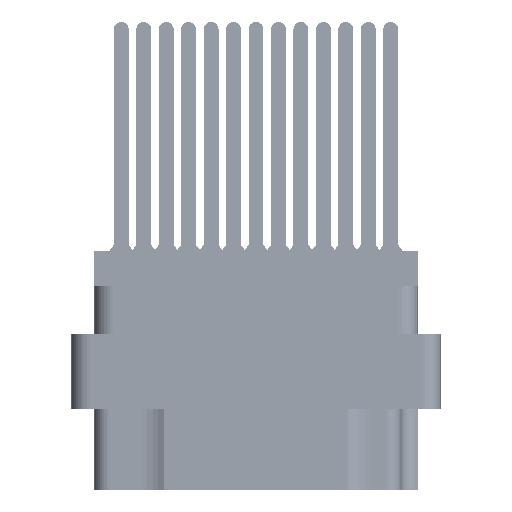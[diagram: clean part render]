
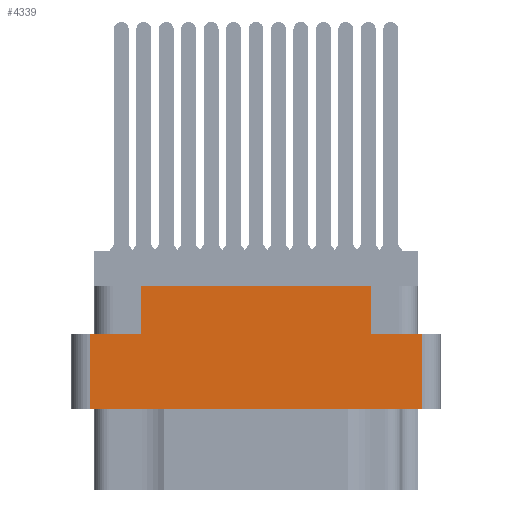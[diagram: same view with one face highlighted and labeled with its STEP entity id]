
A CAD part, left-side view. The second image highlights one B-rep face of the part: STEP entity #4339.
In plain terms, the highlighted planar face has unit normal (-1, 0, 0).
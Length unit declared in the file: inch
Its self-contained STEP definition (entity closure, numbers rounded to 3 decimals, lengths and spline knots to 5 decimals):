
#278 = LINE ( 'NONE', #73736, #49659 ) ;
#703 = EDGE_LOOP ( 'NONE', ( #63365, #63443, #44214, #51385, #26154, #58435, #69929, #70397 ) ) ;
#1515 = LINE ( 'NONE', #16146, #4211 ) ;
#2297 = DIRECTION ( 'NONE',  ( 0., -1., 0. ) ) ;
#3576 = VERTEX_POINT ( 'NONE', #31342 ) ;
#3628 = VECTOR ( 'NONE', #42525, 39.37008 ) ;
#4211 = VECTOR ( 'NONE', #44719, 39.37008 ) ;
#4339 = ADVANCED_FACE ( 'NONE', ( #58785 ), #70136, .T. ) ;
#5164 = CARTESIAN_POINT ( 'NONE',  ( -1.359, -0.555, -0.529 ) ) ;
#6587 = VERTEX_POINT ( 'NONE', #29007 ) ;
#7041 = CARTESIAN_POINT ( 'NONE',  ( -1.359, 0., -0.277 ) ) ;
#16146 = CARTESIAN_POINT ( 'NONE',  ( -1.359, -0.3825, -0.277 ) ) ;
#17005 = CARTESIAN_POINT ( 'NONE',  ( -1.359, -0.555, -0.277 ) ) ;
#17442 = CARTESIAN_POINT ( 'NONE',  ( -1.359, 0., -0.277 ) ) ;
#17492 = AXIS2_PLACEMENT_3D ( 'NONE', #53207, #58219, #24436 ) ;
#19359 = DIRECTION ( 'NONE',  ( 0., -1., 0. ) ) ;
#19883 = VERTEX_POINT ( 'NONE', #41083 ) ;
#20687 = DIRECTION ( 'NONE',  ( 0., 0., 1. ) ) ;
#21098 = VERTEX_POINT ( 'NONE', #5164 ) ;
#22290 = DIRECTION ( 'NONE',  ( 0., 0., -1. ) ) ;
#23563 = VECTOR ( 'NONE', #2297, 39.37008 ) ;
#24436 = DIRECTION ( 'NONE',  ( 0., 0., 1. ) ) ;
#25910 = LINE ( 'NONE', #7041, #54577 ) ;
#26154 = ORIENTED_EDGE ( 'NONE', *, *, #35219, .F. ) ;
#26177 = CARTESIAN_POINT ( 'NONE',  ( -1.359, 0.3825, -0.277 ) ) ;
#26388 = EDGE_CURVE ( 'NONE', #6587, #50143, #278, .T. ) ;
#26515 = CARTESIAN_POINT ( 'NONE',  ( -1.359, -0.555, -0.798 ) ) ;
#26758 = DIRECTION ( 'NONE',  ( 0., 0., 1. ) ) ;
#27767 = EDGE_CURVE ( 'NONE', #21098, #68417, #36043, .T. ) ;
#29007 = CARTESIAN_POINT ( 'NONE',  ( -1.359, 0.3825, -0.117 ) ) ;
#29475 = EDGE_CURVE ( 'NONE', #21098, #19883, #31367, .T. ) ;
#31342 = CARTESIAN_POINT ( 'NONE',  ( -1.359, 0.3825, -0.277 ) ) ;
#31367 = LINE ( 'NONE', #36776, #3628 ) ;
#33068 = CARTESIAN_POINT ( 'NONE',  ( -1.359, -0.3825, -0.117 ) ) ;
#35219 = EDGE_CURVE ( 'NONE', #59432, #68417, #54926, .T. ) ;
#36043 = LINE ( 'NONE', #26515, #62841 ) ;
#36776 = CARTESIAN_POINT ( 'NONE',  ( -1.359, 0., -0.529 ) ) ;
#40243 = CARTESIAN_POINT ( 'NONE',  ( -1.359, 0.555, -0.798 ) ) ;
#40484 = EDGE_CURVE ( 'NONE', #59432, #50143, #1515, .T. ) ;
#41083 = CARTESIAN_POINT ( 'NONE',  ( -1.359, 0.555, -0.529 ) ) ;
#42402 = VECTOR ( 'NONE', #20687, 39.37008 ) ;
#42525 = DIRECTION ( 'NONE',  ( 0., 1., 0. ) ) ;
#44214 = ORIENTED_EDGE ( 'NONE', *, *, #29475, .F. ) ;
#44227 = LINE ( 'NONE', #26177, #42402 ) ;
#44719 = DIRECTION ( 'NONE',  ( 0., 0., 1. ) ) ;
#49659 = VECTOR ( 'NONE', #50353, 39.37008 ) ;
#50143 = VERTEX_POINT ( 'NONE', #33068 ) ;
#50353 = DIRECTION ( 'NONE',  ( 0., -1., 0. ) ) ;
#51385 = ORIENTED_EDGE ( 'NONE', *, *, #27767, .T. ) ;
#53134 = VERTEX_POINT ( 'NONE', #71865 ) ;
#53207 = CARTESIAN_POINT ( 'NONE',  ( -1.359, -0.617, -0.798 ) ) ;
#54577 = VECTOR ( 'NONE', #19359, 39.37008 ) ;
#54926 = LINE ( 'NONE', #17442, #23563 ) ;
#56969 = CARTESIAN_POINT ( 'NONE',  ( -1.359, -0.3825, -0.277 ) ) ;
#58219 = DIRECTION ( 'NONE',  ( -1., 0., 0. ) ) ;
#58435 = ORIENTED_EDGE ( 'NONE', *, *, #40484, .T. ) ;
#58785 = FACE_OUTER_BOUND ( 'NONE', #703, .T. ) ;
#59432 = VERTEX_POINT ( 'NONE', #56969 ) ;
#61421 = VECTOR ( 'NONE', #22290, 39.37008 ) ;
#61870 = EDGE_CURVE ( 'NONE', #53134, #19883, #73798, .T. ) ;
#62841 = VECTOR ( 'NONE', #26758, 39.37008 ) ;
#63365 = ORIENTED_EDGE ( 'NONE', *, *, #68020, .F. ) ;
#63443 = ORIENTED_EDGE ( 'NONE', *, *, #61870, .T. ) ;
#63532 = EDGE_CURVE ( 'NONE', #3576, #6587, #44227, .T. ) ;
#68020 = EDGE_CURVE ( 'NONE', #53134, #3576, #25910, .T. ) ;
#68417 = VERTEX_POINT ( 'NONE', #17005 ) ;
#69929 = ORIENTED_EDGE ( 'NONE', *, *, #26388, .F. ) ;
#70136 = PLANE ( 'NONE',  #17492 ) ;
#70397 = ORIENTED_EDGE ( 'NONE', *, *, #63532, .F. ) ;
#71865 = CARTESIAN_POINT ( 'NONE',  ( -1.359, 0.555, -0.277 ) ) ;
#73736 = CARTESIAN_POINT ( 'NONE',  ( -1.359, 0.617, -0.117 ) ) ;
#73798 = LINE ( 'NONE', #40243, #61421 ) ;
